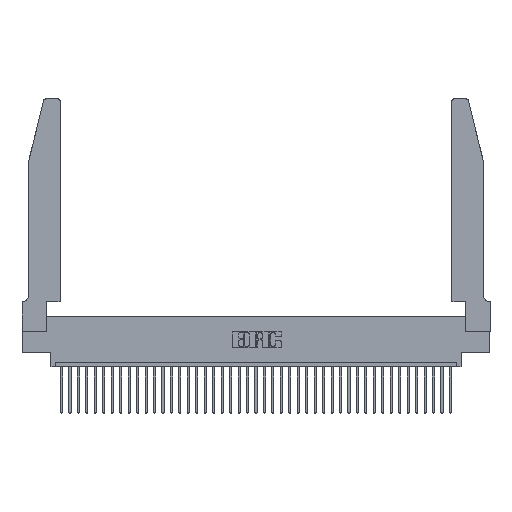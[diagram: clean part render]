
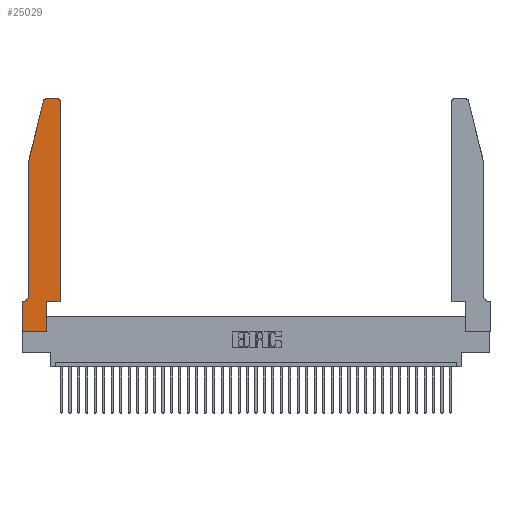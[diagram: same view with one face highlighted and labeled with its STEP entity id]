
A CAD part, top view. The second image highlights one B-rep face of the part: STEP entity #25029.
In plain terms, the highlighted planar face has unit normal (0, 0, 1).
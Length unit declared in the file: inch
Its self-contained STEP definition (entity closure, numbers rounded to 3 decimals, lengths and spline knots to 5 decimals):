
#31 = VECTOR ( 'NONE', #22376, 39.37008 ) ;
#69 = ORIENTED_EDGE ( 'NONE', *, *, #27409, .T. ) ;
#203 = EDGE_CURVE ( 'NONE', #21087, #5376, #33260, .T. ) ;
#243 = CARTESIAN_POINT ( 'NONE',  ( 0.4505, 0.35, 0.37 ) ) ;
#293 = EDGE_CURVE ( 'NONE', #11992, #2943, #12651, .T. ) ;
#510 = ORIENTED_EDGE ( 'NONE', *, *, #2013, .T. ) ;
#727 = VECTOR ( 'NONE', #8315, 39.37008 ) ;
#1251 = CARTESIAN_POINT ( 'NONE',  ( 0.2865, 0.35, 0.37 ) ) ;
#1432 = DIRECTION ( 'NONE',  ( -1., 0., 0. ) ) ;
#2013 = EDGE_CURVE ( 'NONE', #2943, #18868, #13951, .T. ) ;
#2826 = VERTEX_POINT ( 'NONE', #37478 ) ;
#2943 = VERTEX_POINT ( 'NONE', #21766 ) ;
#3549 = VECTOR ( 'NONE', #36427, 39.37008 ) ;
#3865 = DIRECTION ( 'NONE',  ( 0., -1., 0. ) ) ;
#5044 = ORIENTED_EDGE ( 'NONE', *, *, #22263, .T. ) ;
#5068 = CARTESIAN_POINT ( 'NONE',  ( 0., 0., 0.37 ) ) ;
#5376 = VERTEX_POINT ( 'NONE', #38344 ) ;
#5401 = ORIENTED_EDGE ( 'NONE', *, *, #27988, .T. ) ;
#5982 = VECTOR ( 'NONE', #3865, 39.37008 ) ;
#6144 = CARTESIAN_POINT ( 'NONE',  ( 0.4505, 0.35, 0.37 ) ) ;
#6895 = CARTESIAN_POINT ( 'NONE',  ( 0.2865, 0.35, 0.37 ) ) ;
#6977 = AXIS2_PLACEMENT_3D ( 'NONE', #38233, #23123, #8168 ) ;
#7944 = LINE ( 'NONE', #5068, #727 ) ;
#8168 = DIRECTION ( 'NONE',  ( -1., 0., 0. ) ) ;
#8238 = LINE ( 'NONE', #31698, #18735 ) ;
#8315 = DIRECTION ( 'NONE',  ( 0., -1., 0. ) ) ;
#9209 = ORIENTED_EDGE ( 'NONE', *, *, #13133, .T. ) ;
#9244 = VERTEX_POINT ( 'NONE', #12664 ) ;
#9762 = CARTESIAN_POINT ( 'NONE',  ( 0.0755, 2., 0.37 ) ) ;
#10128 = EDGE_LOOP ( 'NONE', ( #37373, #510, #18986, #9209, #69, #5401, #24189, #13053, #13253, #32582, #5044, #15837 ) ) ;
#10791 = VECTOR ( 'NONE', #24791, 39.37008 ) ;
#11992 = VERTEX_POINT ( 'NONE', #17041 ) ;
#12651 = LINE ( 'NONE', #27474, #19808 ) ;
#12664 = CARTESIAN_POINT ( 'NONE',  ( 0.4505, 0.35, 0.37 ) ) ;
#12691 = DIRECTION ( 'NONE',  ( 1., 0., 0. ) ) ;
#13053 = ORIENTED_EDGE ( 'NONE', *, *, #203, .T. ) ;
#13133 = EDGE_CURVE ( 'NONE', #33906, #31091, #37051, .T. ) ;
#13253 = ORIENTED_EDGE ( 'NONE', *, *, #23510, .T. ) ;
#13951 = CIRCLE ( 'NONE', #29223, 0.03 ) ;
#14521 = EDGE_CURVE ( 'NONE', #16388, #9244, #31207, .T. ) ;
#15454 = LINE ( 'NONE', #25577, #36510 ) ;
#15813 = DIRECTION ( 'NONE',  ( 1., 0., 0. ) ) ;
#15837 = ORIENTED_EDGE ( 'NONE', *, *, #17281, .T. ) ;
#15889 = CARTESIAN_POINT ( 'NONE',  ( 0.0755, 2., 0.37 ) ) ;
#16388 = VERTEX_POINT ( 'NONE', #1251 ) ;
#16586 = EDGE_CURVE ( 'NONE', #18868, #33906, #15454, .T. ) ;
#17041 = CARTESIAN_POINT ( 'NONE',  ( 0.4205, 2.75, 0.37 ) ) ;
#17281 = EDGE_CURVE ( 'NONE', #34795, #11992, #25928, .T. ) ;
#17840 = CARTESIAN_POINT ( 'NONE',  ( 0., 0., 0.37 ) ) ;
#18409 = LINE ( 'NONE', #243, #10791 ) ;
#18735 = VECTOR ( 'NONE', #1432, 39.37008 ) ;
#18868 = VERTEX_POINT ( 'NONE', #25676 ) ;
#18986 = ORIENTED_EDGE ( 'NONE', *, *, #16586, .T. ) ;
#19271 = CIRCLE ( 'NONE', #6977, 0.07 ) ;
#19808 = VECTOR ( 'NONE', #37075, 39.37008 ) ;
#21040 = CARTESIAN_POINT ( 'NONE',  ( 0.4205, 2.72, 0.37 ) ) ;
#21087 = VERTEX_POINT ( 'NONE', #37915 ) ;
#21766 = CARTESIAN_POINT ( 'NONE',  ( 0.284, 2.75, 0.37 ) ) ;
#22263 = EDGE_CURVE ( 'NONE', #9244, #34795, #18409, .T. ) ;
#22376 = DIRECTION ( 'NONE',  ( 0., 1., 0. ) ) ;
#22970 = LINE ( 'NONE', #6895, #31 ) ;
#23123 = DIRECTION ( 'NONE',  ( 0., 0., -1. ) ) ;
#23510 = EDGE_CURVE ( 'NONE', #5376, #16388, #22970, .T. ) ;
#24189 = ORIENTED_EDGE ( 'NONE', *, *, #35945, .T. ) ;
#24791 = DIRECTION ( 'NONE',  ( 0., 1., 0. ) ) ;
#25029 = ADVANCED_FACE ( 'NONE', ( #36229 ), #34184, .T. ) ;
#25448 = DIRECTION ( 'NONE',  ( -0.239, -0.971, 0. ) ) ;
#25462 = DIRECTION ( 'NONE',  ( 0., 0., 1. ) ) ;
#25577 = CARTESIAN_POINT ( 'NONE',  ( 0.0755, 2., 0.37 ) ) ;
#25676 = CARTESIAN_POINT ( 'NONE',  ( 0.25487, 2.72718, 0.37 ) ) ;
#25928 = CIRCLE ( 'NONE', #37356, 0.03 ) ;
#25989 = DIRECTION ( 'NONE',  ( 1., 0., 0. ) ) ;
#26836 = CARTESIAN_POINT ( 'NONE',  ( 0.0055, 0.35, 0.37 ) ) ;
#27409 = EDGE_CURVE ( 'NONE', #31091, #38395, #19271, .T. ) ;
#27474 = CARTESIAN_POINT ( 'NONE',  ( 0.2605, 2.75, 0.37 ) ) ;
#27988 = EDGE_CURVE ( 'NONE', #38395, #2826, #8238, .T. ) ;
#28423 = CARTESIAN_POINT ( 'NONE',  ( 0., 0.35, 0.37 ) ) ;
#29070 = CARTESIAN_POINT ( 'NONE',  ( 0.284, 2.72, 0.37 ) ) ;
#29223 = AXIS2_PLACEMENT_3D ( 'NONE', #29070, #25462, #25989 ) ;
#30285 = CARTESIAN_POINT ( 'NONE',  ( 0.4505, 2.72, 0.37 ) ) ;
#30715 = DIRECTION ( 'NONE',  ( 0., 0., 1. ) ) ;
#31091 = VERTEX_POINT ( 'NONE', #33835 ) ;
#31207 = LINE ( 'NONE', #6144, #35031 ) ;
#31698 = CARTESIAN_POINT ( 'NONE',  ( 0.0755, 0.35, 0.37 ) ) ;
#32582 = ORIENTED_EDGE ( 'NONE', *, *, #14521, .T. ) ;
#33260 = LINE ( 'NONE', #17840, #3549 ) ;
#33835 = CARTESIAN_POINT ( 'NONE',  ( 0.0755, 0.42, 0.37 ) ) ;
#33906 = VERTEX_POINT ( 'NONE', #9762 ) ;
#34184 = PLANE ( 'NONE',  #34504 ) ;
#34504 = AXIS2_PLACEMENT_3D ( 'NONE', #28423, #37506, #15813 ) ;
#34795 = VERTEX_POINT ( 'NONE', #30285 ) ;
#35031 = VECTOR ( 'NONE', #12691, 39.37008 ) ;
#35945 = EDGE_CURVE ( 'NONE', #2826, #21087, #7944, .T. ) ;
#36229 = FACE_OUTER_BOUND ( 'NONE', #10128, .T. ) ;
#36427 = DIRECTION ( 'NONE',  ( 1., 0., 0. ) ) ;
#36510 = VECTOR ( 'NONE', #25448, 39.37008 ) ;
#36575 = DIRECTION ( 'NONE',  ( 1., 0., 0. ) ) ;
#37051 = LINE ( 'NONE', #15889, #5982 ) ;
#37075 = DIRECTION ( 'NONE',  ( -1., 0., 0. ) ) ;
#37356 = AXIS2_PLACEMENT_3D ( 'NONE', #21040, #30715, #36575 ) ;
#37373 = ORIENTED_EDGE ( 'NONE', *, *, #293, .T. ) ;
#37478 = CARTESIAN_POINT ( 'NONE',  ( 0., 0.35, 0.37 ) ) ;
#37506 = DIRECTION ( 'NONE',  ( 0., 0., 1. ) ) ;
#37915 = CARTESIAN_POINT ( 'NONE',  ( 0., 0., 0.37 ) ) ;
#38233 = CARTESIAN_POINT ( 'NONE',  ( 0.0055, 0.42, 0.37 ) ) ;
#38344 = CARTESIAN_POINT ( 'NONE',  ( 0.2865, 0., 0.37 ) ) ;
#38395 = VERTEX_POINT ( 'NONE', #26836 ) ;
